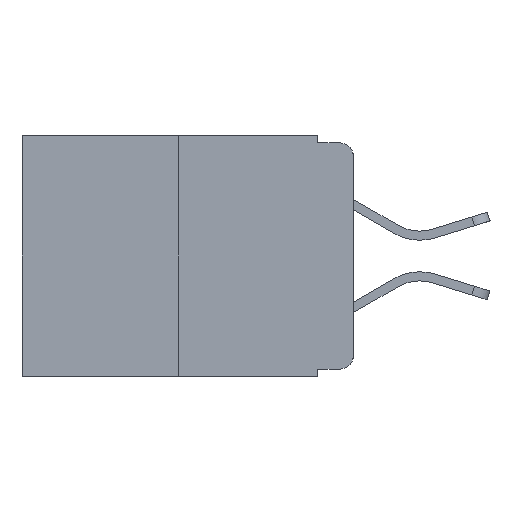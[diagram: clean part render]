
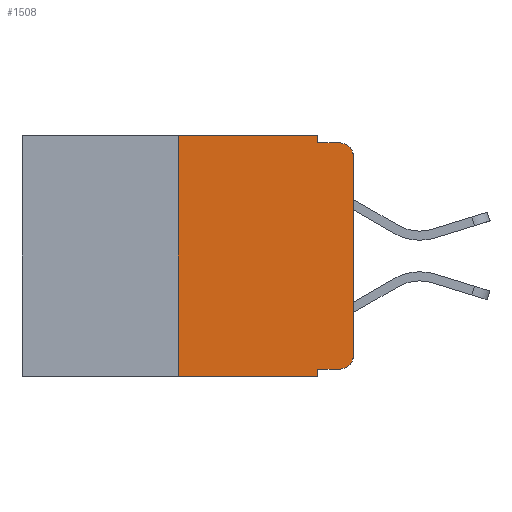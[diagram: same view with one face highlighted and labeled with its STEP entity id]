
A CAD part, left-side view. The second image highlights one B-rep face of the part: STEP entity #1508.
In plain terms, the highlighted planar face has unit normal (-1, 0, 0).
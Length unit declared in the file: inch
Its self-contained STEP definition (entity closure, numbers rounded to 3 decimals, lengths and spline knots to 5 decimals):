
#48 = DIRECTION ( 'NONE',  ( 1., 0., 0. ) ) ;
#453 = CARTESIAN_POINT ( 'NONE',  ( 0., 0., -0.03 ) ) ;
#1507 = VERTEX_POINT ( 'NONE', #21791 ) ;
#1508 = ADVANCED_FACE ( 'NONE', ( #17031 ), #1934, .F. ) ;
#1934 = PLANE ( 'NONE',  #20884 ) ;
#2395 = ORIENTED_EDGE ( 'NONE', *, *, #12601, .F. ) ;
#2594 = CARTESIAN_POINT ( 'NONE',  ( 0., 0.02, -0.01 ) ) ;
#2779 = DIRECTION ( 'NONE',  ( 0., 0., -1. ) ) ;
#2797 = CARTESIAN_POINT ( 'NONE',  ( 0., 0.051, -0.333 ) ) ;
#3203 = DIRECTION ( 'NONE',  ( 0., 0., -1. ) ) ;
#3386 = EDGE_LOOP ( 'NONE', ( #21717, #14223, #6593, #7713, #2395, #20737, #9933, #19962, #8969, #9296 ) ) ;
#3917 = CARTESIAN_POINT ( 'NONE',  ( 0., 0.051, -0.01 ) ) ;
#4246 = DIRECTION ( 'NONE',  ( 0., -1., 0. ) ) ;
#4525 = CARTESIAN_POINT ( 'NONE',  ( 0., 0.051, 0. ) ) ;
#4625 = EDGE_CURVE ( 'NONE', #4936, #5120, #15292, .T. ) ;
#4906 = EDGE_CURVE ( 'NONE', #15018, #8468, #14708, .T. ) ;
#4936 = VERTEX_POINT ( 'NONE', #3917 ) ;
#5033 = CARTESIAN_POINT ( 'NONE',  ( 0., 0.051, 0. ) ) ;
#5120 = VERTEX_POINT ( 'NONE', #2594 ) ;
#5319 = VECTOR ( 'NONE', #13605, 39.37008 ) ;
#6310 = LINE ( 'NONE', #9419, #8861 ) ;
#6463 = CIRCLE ( 'NONE', #20532, 0.02 ) ;
#6593 = ORIENTED_EDGE ( 'NONE', *, *, #4625, .F. ) ;
#7011 = DIRECTION ( 'NONE',  ( 0., 0., -1. ) ) ;
#7713 = ORIENTED_EDGE ( 'NONE', *, *, #11360, .F. ) ;
#8468 = VERTEX_POINT ( 'NONE', #453 ) ;
#8573 = CARTESIAN_POINT ( 'NONE',  ( 0., 0.473, 0. ) ) ;
#8861 = VECTOR ( 'NONE', #2779, 39.37008 ) ;
#8969 = ORIENTED_EDGE ( 'NONE', *, *, #18081, .T. ) ;
#8976 = VECTOR ( 'NONE', #4246, 39.37008 ) ;
#9007 = VECTOR ( 'NONE', #19780, 39.37008 ) ;
#9114 = LINE ( 'NONE', #9545, #8976 ) ;
#9296 = ORIENTED_EDGE ( 'NONE', *, *, #17269, .T. ) ;
#9419 = CARTESIAN_POINT ( 'NONE',  ( 0., 0.051, 0. ) ) ;
#9545 = CARTESIAN_POINT ( 'NONE',  ( 0., 0.051, -0.333 ) ) ;
#9910 = AXIS2_PLACEMENT_3D ( 'NONE', #10233, #20555, #15576 ) ;
#9933 = ORIENTED_EDGE ( 'NONE', *, *, #10568, .T. ) ;
#10233 = CARTESIAN_POINT ( 'NONE',  ( 0., 0.02, -0.03 ) ) ;
#10568 = EDGE_CURVE ( 'NONE', #1507, #16171, #11337, .T. ) ;
#10569 = EDGE_CURVE ( 'NONE', #1507, #20643, #14719, .T. ) ;
#11273 = CARTESIAN_POINT ( 'NONE',  ( 0., 0.02, -0.313 ) ) ;
#11337 = LINE ( 'NONE', #21561, #13368 ) ;
#11360 = EDGE_CURVE ( 'NONE', #11949, #4936, #19292, .T. ) ;
#11949 = VERTEX_POINT ( 'NONE', #5033 ) ;
#12162 = EDGE_CURVE ( 'NONE', #8468, #5120, #13750, .T. ) ;
#12601 = EDGE_CURVE ( 'NONE', #20643, #11949, #15230, .T. ) ;
#12990 = CARTESIAN_POINT ( 'NONE',  ( 0., 0.25, 0. ) ) ;
#13081 = CARTESIAN_POINT ( 'NONE',  ( 0., 0., 0. ) ) ;
#13368 = VECTOR ( 'NONE', #21456, 39.37008 ) ;
#13605 = DIRECTION ( 'NONE',  ( 0., -1., 0. ) ) ;
#13718 = VECTOR ( 'NONE', #16369, 39.37008 ) ;
#13750 = CIRCLE ( 'NONE', #9910, 0.02 ) ;
#13993 = EDGE_CURVE ( 'NONE', #18025, #16171, #6310, .T. ) ;
#14223 = ORIENTED_EDGE ( 'NONE', *, *, #12162, .T. ) ;
#14708 = LINE ( 'NONE', #13081, #9007 ) ;
#14719 = LINE ( 'NONE', #12990, #13718 ) ;
#15018 = VERTEX_POINT ( 'NONE', #21026 ) ;
#15230 = LINE ( 'NONE', #16796, #5319 ) ;
#15292 = LINE ( 'NONE', #18514, #16012 ) ;
#15444 = VERTEX_POINT ( 'NONE', #19340 ) ;
#15469 = VECTOR ( 'NONE', #19606, 39.37008 ) ;
#15576 = DIRECTION ( 'NONE',  ( 0., 0., -1. ) ) ;
#16012 = VECTOR ( 'NONE', #20053, 39.37008 ) ;
#16171 = VERTEX_POINT ( 'NONE', #19039 ) ;
#16369 = DIRECTION ( 'NONE',  ( 0., 0., 1. ) ) ;
#16796 = CARTESIAN_POINT ( 'NONE',  ( 0., 0.473, 0. ) ) ;
#16942 = CARTESIAN_POINT ( 'NONE',  ( 0., 0.25, 0. ) ) ;
#17031 = FACE_OUTER_BOUND ( 'NONE', #3386, .T. ) ;
#17269 = EDGE_CURVE ( 'NONE', #15444, #15018, #6463, .T. ) ;
#18025 = VERTEX_POINT ( 'NONE', #2797 ) ;
#18081 = EDGE_CURVE ( 'NONE', #18025, #15444, #9114, .T. ) ;
#18514 = CARTESIAN_POINT ( 'NONE',  ( 0., 0.051, -0.01 ) ) ;
#19039 = CARTESIAN_POINT ( 'NONE',  ( 0., 0.051, -0.343 ) ) ;
#19292 = LINE ( 'NONE', #4525, #15469 ) ;
#19340 = CARTESIAN_POINT ( 'NONE',  ( 0., 0.02, -0.333 ) ) ;
#19606 = DIRECTION ( 'NONE',  ( 0., 0., -1. ) ) ;
#19780 = DIRECTION ( 'NONE',  ( 0., 0., 1. ) ) ;
#19828 = DIRECTION ( 'NONE',  ( -1., 0., 0. ) ) ;
#19962 = ORIENTED_EDGE ( 'NONE', *, *, #13993, .F. ) ;
#20053 = DIRECTION ( 'NONE',  ( 0., -1., 0. ) ) ;
#20532 = AXIS2_PLACEMENT_3D ( 'NONE', #11273, #19828, #3203 ) ;
#20555 = DIRECTION ( 'NONE',  ( -1., 0., 0. ) ) ;
#20643 = VERTEX_POINT ( 'NONE', #16942 ) ;
#20737 = ORIENTED_EDGE ( 'NONE', *, *, #10569, .F. ) ;
#20884 = AXIS2_PLACEMENT_3D ( 'NONE', #8573, #48, #7011 ) ;
#21026 = CARTESIAN_POINT ( 'NONE',  ( 0., 0., -0.313 ) ) ;
#21456 = DIRECTION ( 'NONE',  ( 0., -1., 0. ) ) ;
#21561 = CARTESIAN_POINT ( 'NONE',  ( 0., 0.473, -0.343 ) ) ;
#21717 = ORIENTED_EDGE ( 'NONE', *, *, #4906, .T. ) ;
#21791 = CARTESIAN_POINT ( 'NONE',  ( 0., 0.25, -0.343 ) ) ;
